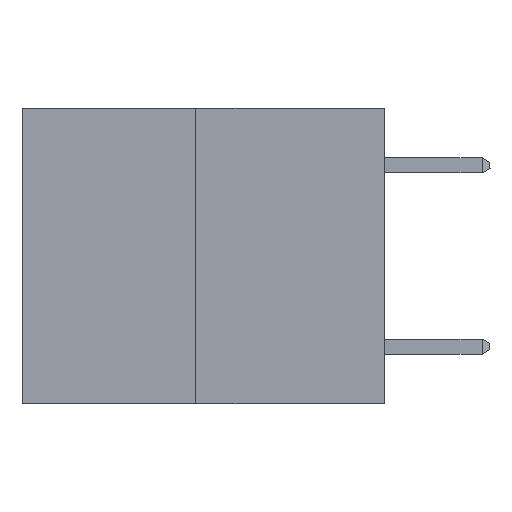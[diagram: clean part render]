
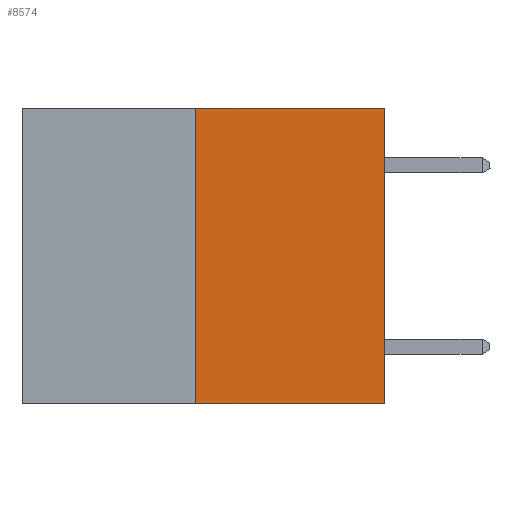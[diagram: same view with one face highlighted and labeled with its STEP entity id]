
A CAD part, left-side view. The second image highlights one B-rep face of the part: STEP entity #8574.
In plain terms, the highlighted planar face has unit normal (-1, 0, 0).
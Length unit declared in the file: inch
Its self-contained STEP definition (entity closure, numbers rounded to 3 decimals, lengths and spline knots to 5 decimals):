
#569 = LINE ( 'NONE', #11639, #18805 ) ;
#810 = ORIENTED_EDGE ( 'NONE', *, *, #3858, .T. ) ;
#870 = CARTESIAN_POINT ( 'NONE',  ( 0., 0.312, -0.49 ) ) ;
#1288 = FACE_OUTER_BOUND ( 'NONE', #13149, .T. ) ;
#2535 = DIRECTION ( 'NONE',  ( 0., 0., 1. ) ) ;
#2707 = DIRECTION ( 'NONE',  ( 0., -1., 0. ) ) ;
#3858 = EDGE_CURVE ( 'NONE', #12125, #13753, #9440, .T. ) ;
#4169 = CARTESIAN_POINT ( 'NONE',  ( 0., 0.312, -0.49 ) ) ;
#4227 = CARTESIAN_POINT ( 'NONE',  ( 0., 0.6, 0. ) ) ;
#4583 = EDGE_CURVE ( 'NONE', #12125, #9841, #18021, .T. ) ;
#6440 = ORIENTED_EDGE ( 'NONE', *, *, #4583, .F. ) ;
#6676 = DIRECTION ( 'NONE',  ( 0., 0., -1. ) ) ;
#6997 = CARTESIAN_POINT ( 'NONE',  ( 0., 0.6, 0. ) ) ;
#8574 = ADVANCED_FACE ( 'NONE', ( #1288 ), #17666, .F. ) ;
#9440 = LINE ( 'NONE', #18937, #18887 ) ;
#9841 = VERTEX_POINT ( 'NONE', #14172 ) ;
#9961 = LINE ( 'NONE', #4227, #20282 ) ;
#10484 = EDGE_CURVE ( 'NONE', #13753, #14802, #569, .T. ) ;
#10731 = CARTESIAN_POINT ( 'NONE',  ( 0., 0., -0.49 ) ) ;
#10794 = EDGE_CURVE ( 'NONE', #9841, #14802, #9961, .T. ) ;
#11639 = CARTESIAN_POINT ( 'NONE',  ( 0., 0., 0. ) ) ;
#12125 = VERTEX_POINT ( 'NONE', #870 ) ;
#12542 = DIRECTION ( 'NONE',  ( 1., 0., 0. ) ) ;
#13149 = EDGE_LOOP ( 'NONE', ( #6440, #810, #16904, #18304 ) ) ;
#13753 = VERTEX_POINT ( 'NONE', #10731 ) ;
#14172 = CARTESIAN_POINT ( 'NONE',  ( 0., 0.312, 0. ) ) ;
#14519 = AXIS2_PLACEMENT_3D ( 'NONE', #6997, #12542, #6676 ) ;
#14802 = VERTEX_POINT ( 'NONE', #20509 ) ;
#16904 = ORIENTED_EDGE ( 'NONE', *, *, #10484, .T. ) ;
#17593 = DIRECTION ( 'NONE',  ( 0., -1., 0. ) ) ;
#17666 = PLANE ( 'NONE',  #14519 ) ;
#18021 = LINE ( 'NONE', #4169, #19735 ) ;
#18304 = ORIENTED_EDGE ( 'NONE', *, *, #10794, .F. ) ;
#18805 = VECTOR ( 'NONE', #19541, 39.37008 ) ;
#18887 = VECTOR ( 'NONE', #17593, 39.37008 ) ;
#18937 = CARTESIAN_POINT ( 'NONE',  ( 0., 0.6, -0.49 ) ) ;
#19541 = DIRECTION ( 'NONE',  ( 0., 0., 1. ) ) ;
#19735 = VECTOR ( 'NONE', #2535, 39.37008 ) ;
#20282 = VECTOR ( 'NONE', #2707, 39.37008 ) ;
#20509 = CARTESIAN_POINT ( 'NONE',  ( 0., 0., 0. ) ) ;
